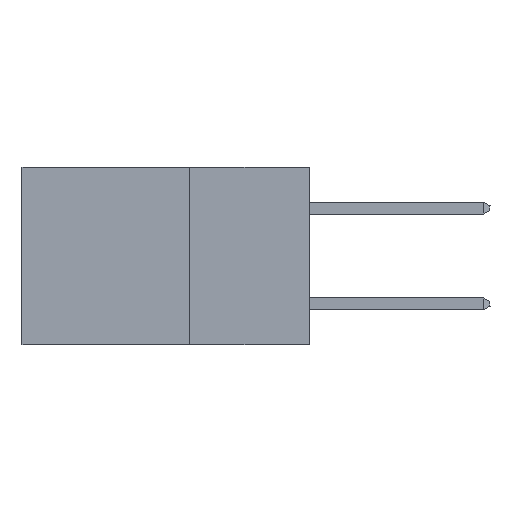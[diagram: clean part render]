
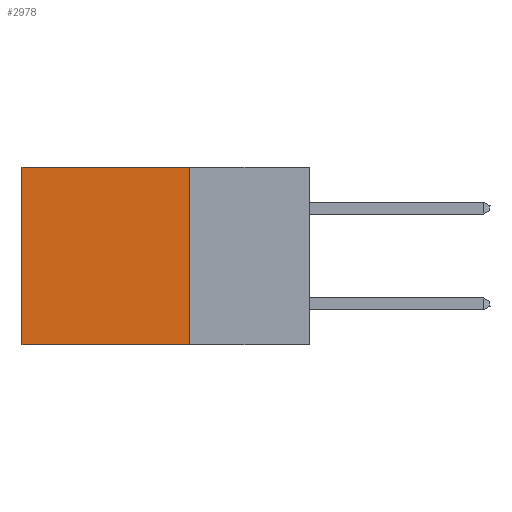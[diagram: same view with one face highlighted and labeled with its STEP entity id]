
A CAD part, left-side view. The second image highlights one B-rep face of the part: STEP entity #2978.
In plain terms, the highlighted planar face has unit normal (-1, 0, 0).
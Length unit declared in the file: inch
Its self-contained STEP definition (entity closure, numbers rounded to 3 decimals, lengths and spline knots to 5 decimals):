
#807 = VECTOR ( 'NONE', #17425, 39.37008 ) ;
#2949 = VERTEX_POINT ( 'NONE', #11560 ) ;
#2978 = ADVANCED_FACE ( 'NONE', ( #5589 ), #18927, .F. ) ;
#4885 = EDGE_CURVE ( 'NONE', #2949, #18594, #28969, .T. ) ;
#5524 = DIRECTION ( 'NONE',  ( 0., 0., -1. ) ) ;
#5589 = FACE_OUTER_BOUND ( 'NONE', #21718, .T. ) ;
#5786 = LINE ( 'NONE', #10216, #18651 ) ;
#7184 = ORIENTED_EDGE ( 'NONE', *, *, #4885, .F. ) ;
#7546 = EDGE_CURVE ( 'NONE', #2949, #21923, #28418, .T. ) ;
#9222 = ORIENTED_EDGE ( 'NONE', *, *, #7546, .T. ) ;
#10216 = CARTESIAN_POINT ( 'NONE',  ( 0.2875, 0.6, 0. ) ) ;
#10484 = DIRECTION ( 'NONE',  ( 0., 0., -1. ) ) ;
#11560 = CARTESIAN_POINT ( 'NONE',  ( 0.2875, 0.25, 0. ) ) ;
#12739 = AXIS2_PLACEMENT_3D ( 'NONE', #15561, #19059, #16074 ) ;
#12824 = ORIENTED_EDGE ( 'NONE', *, *, #21774, .T. ) ;
#13213 = VECTOR ( 'NONE', #10484, 39.37008 ) ;
#14691 = EDGE_CURVE ( 'NONE', #18594, #21493, #17376, .T. ) ;
#15468 = ORIENTED_EDGE ( 'NONE', *, *, #14691, .F. ) ;
#15561 = CARTESIAN_POINT ( 'NONE',  ( 0.2875, 0.25, 0. ) ) ;
#16074 = DIRECTION ( 'NONE',  ( 0., 0., -1. ) ) ;
#17222 = CARTESIAN_POINT ( 'NONE',  ( 0.2875, 0.25, 0. ) ) ;
#17376 = LINE ( 'NONE', #19593, #807 ) ;
#17425 = DIRECTION ( 'NONE',  ( 0., 1., 0. ) ) ;
#18594 = VERTEX_POINT ( 'NONE', #22791 ) ;
#18651 = VECTOR ( 'NONE', #5524, 39.37008 ) ;
#18927 = PLANE ( 'NONE',  #12739 ) ;
#19059 = DIRECTION ( 'NONE',  ( 1., 0., 0. ) ) ;
#19593 = CARTESIAN_POINT ( 'NONE',  ( 0.2875, 0.25, -0.37 ) ) ;
#19707 = CARTESIAN_POINT ( 'NONE',  ( 0.2875, 0.6, 0. ) ) ;
#21493 = VERTEX_POINT ( 'NONE', #23124 ) ;
#21718 = EDGE_LOOP ( 'NONE', ( #12824, #15468, #7184, #9222 ) ) ;
#21774 = EDGE_CURVE ( 'NONE', #21923, #21493, #5786, .T. ) ;
#21923 = VERTEX_POINT ( 'NONE', #19707 ) ;
#21961 = VECTOR ( 'NONE', #23269, 39.37008 ) ;
#22791 = CARTESIAN_POINT ( 'NONE',  ( 0.2875, 0.25, -0.37 ) ) ;
#23124 = CARTESIAN_POINT ( 'NONE',  ( 0.2875, 0.6, -0.37 ) ) ;
#23269 = DIRECTION ( 'NONE',  ( 0., 1., 0. ) ) ;
#25270 = CARTESIAN_POINT ( 'NONE',  ( 0.2875, 0.25, 0. ) ) ;
#28418 = LINE ( 'NONE', #25270, #21961 ) ;
#28969 = LINE ( 'NONE', #17222, #13213 ) ;
